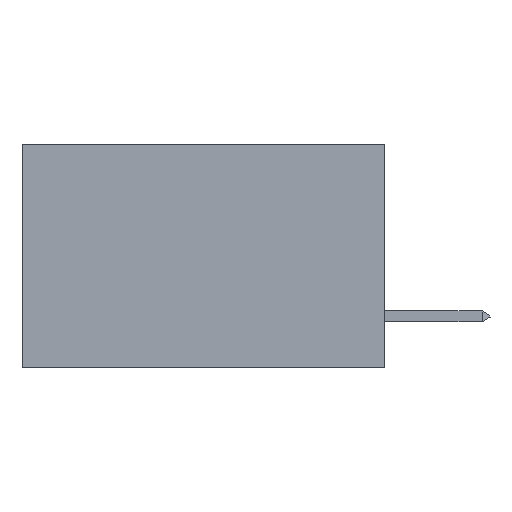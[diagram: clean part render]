
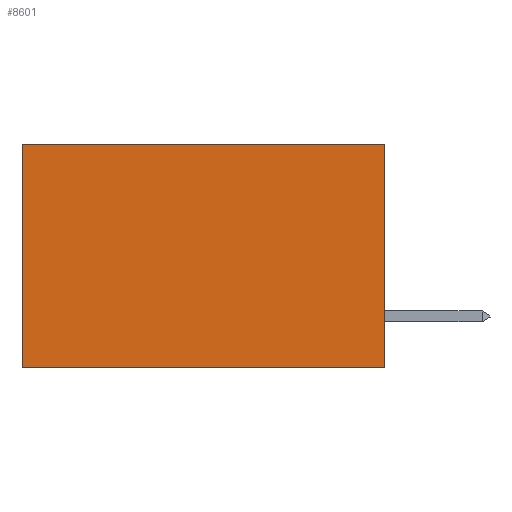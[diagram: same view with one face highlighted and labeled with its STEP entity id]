
A CAD part, left-side view. The second image highlights one B-rep face of the part: STEP entity #8601.
In plain terms, the highlighted planar face has unit normal (-1, 0, 0).
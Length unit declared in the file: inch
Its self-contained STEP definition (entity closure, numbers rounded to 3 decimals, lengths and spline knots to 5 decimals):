
#202 = VECTOR ( 'NONE', #9548, 39.37008 ) ;
#211 = FACE_OUTER_BOUND ( 'NONE', #3078, .T. ) ;
#281 = VERTEX_POINT ( 'NONE', #9674 ) ;
#331 = CARTESIAN_POINT ( 'NONE',  ( 0.2875, 0., -0.37 ) ) ;
#495 = AXIS2_PLACEMENT_3D ( 'NONE', #7643, #2015, #3479 ) ;
#709 = CARTESIAN_POINT ( 'NONE',  ( 0.2875, 0.6, -0.37 ) ) ;
#1677 = DIRECTION ( 'NONE',  ( 0., 0., -1. ) ) ;
#1727 = LINE ( 'NONE', #331, #6088 ) ;
#1830 = ORIENTED_EDGE ( 'NONE', *, *, #4413, .T. ) ;
#1927 = VERTEX_POINT ( 'NONE', #709 ) ;
#2015 = DIRECTION ( 'NONE',  ( 1., 0., 0. ) ) ;
#2806 = CARTESIAN_POINT ( 'NONE',  ( 0.2875, 0.6, 0. ) ) ;
#3078 = EDGE_LOOP ( 'NONE', ( #1830, #4804, #8212, #7182 ) ) ;
#3479 = DIRECTION ( 'NONE',  ( 0., 0., -1. ) ) ;
#3577 = EDGE_CURVE ( 'NONE', #4089, #3737, #8858, .T. ) ;
#3578 = DIRECTION ( 'NONE',  ( 0., 0., -1. ) ) ;
#3612 = CARTESIAN_POINT ( 'NONE',  ( 0.2875, 0., 0. ) ) ;
#3737 = VERTEX_POINT ( 'NONE', #9763 ) ;
#4089 = VERTEX_POINT ( 'NONE', #7706 ) ;
#4413 = EDGE_CURVE ( 'NONE', #3737, #1927, #6501, .T. ) ;
#4520 = VECTOR ( 'NONE', #3578, 39.37008 ) ;
#4713 = EDGE_CURVE ( 'NONE', #4089, #281, #4750, .T. ) ;
#4750 = LINE ( 'NONE', #5473, #7279 ) ;
#4804 = ORIENTED_EDGE ( 'NONE', *, *, #6839, .F. ) ;
#5473 = CARTESIAN_POINT ( 'NONE',  ( 0.2875, 0., 0. ) ) ;
#6088 = VECTOR ( 'NONE', #6265, 39.37008 ) ;
#6265 = DIRECTION ( 'NONE',  ( 0., 1., 0. ) ) ;
#6501 = LINE ( 'NONE', #2806, #4520 ) ;
#6839 = EDGE_CURVE ( 'NONE', #281, #1927, #1727, .T. ) ;
#7182 = ORIENTED_EDGE ( 'NONE', *, *, #3577, .T. ) ;
#7279 = VECTOR ( 'NONE', #1677, 39.37008 ) ;
#7643 = CARTESIAN_POINT ( 'NONE',  ( 0.2875, 0., 0. ) ) ;
#7706 = CARTESIAN_POINT ( 'NONE',  ( 0.2875, 0., 0. ) ) ;
#8212 = ORIENTED_EDGE ( 'NONE', *, *, #4713, .F. ) ;
#8601 = ADVANCED_FACE ( 'NONE', ( #211 ), #8861, .F. ) ;
#8858 = LINE ( 'NONE', #3612, #202 ) ;
#8861 = PLANE ( 'NONE',  #495 ) ;
#9548 = DIRECTION ( 'NONE',  ( 0., 1., 0. ) ) ;
#9674 = CARTESIAN_POINT ( 'NONE',  ( 0.2875, 0., -0.37 ) ) ;
#9763 = CARTESIAN_POINT ( 'NONE',  ( 0.2875, 0.6, 0. ) ) ;
